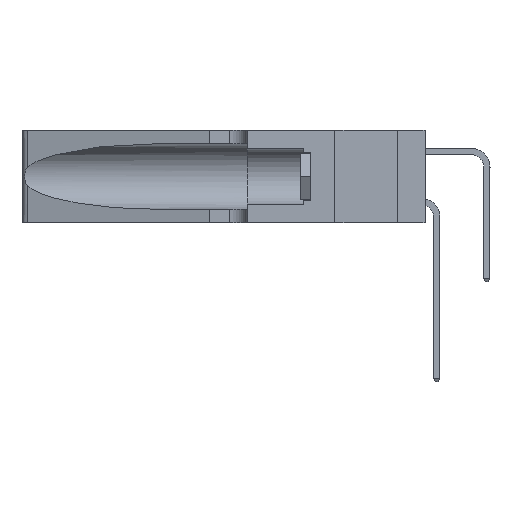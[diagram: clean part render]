
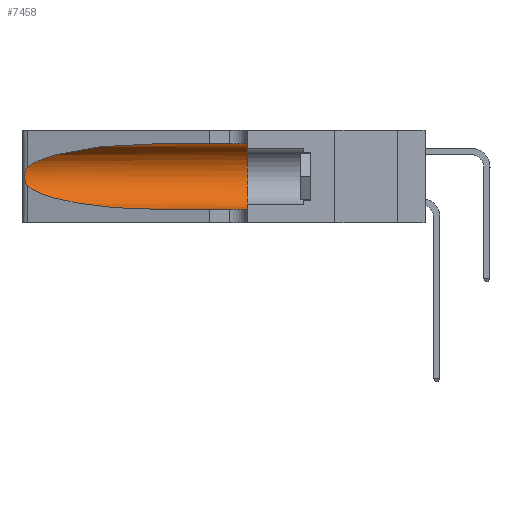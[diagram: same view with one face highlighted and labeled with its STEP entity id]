
A CAD part, left-side view. The second image highlights one B-rep face of the part: STEP entity #7458.
In plain terms, the highlighted cylindrical face has radius 3.308 mm (diameter 6.617 mm), a partial arc.
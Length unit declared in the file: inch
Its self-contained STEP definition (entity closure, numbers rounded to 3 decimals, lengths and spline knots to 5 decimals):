
#196 = AXIS2_PLACEMENT_3D ( 'NONE', #17155, #12661, #23664 ) ;
#1073 = ORIENTED_EDGE ( 'NONE', *, *, #27238, .T. ) ;
#1272 = CARTESIAN_POINT ( 'NONE',  ( 0.1305, 0.72297, 0.05475 ) ) ;
#1434 = LINE ( 'NONE', #25243, #9130 ) ;
#2066 = CARTESIAN_POINT ( 'NONE',  ( 0.25856, 1.23593, 0.16098 ) ) ;
#2228 =( BOUNDED_CURVE ( )  B_SPLINE_CURVE ( 3, ( #24379, #26508, #22404, #5308 ),
 .UNSPECIFIED., .F., .F. ) 
 B_SPLINE_CURVE_WITH_KNOTS ( ( 4, 4 ),
 ( 1.5708, 2.84003 ),
 .UNSPECIFIED. ) 
 CURVE ( )  GEOMETRIC_REPRESENTATION_ITEM ( )  RATIONAL_B_SPLINE_CURVE ( ( 1., 0.87, 0.87, 1. ) ) 
 REPRESENTATION_ITEM ( '' )  );
#2987 = CARTESIAN_POINT ( 'NONE',  ( 0.18966, 0.96281, 0.05475 ) ) ;
#3248 = CARTESIAN_POINT ( 'NONE',  ( 0.1305, 0.72297, 0.31525 ) ) ;
#3663 = ORIENTED_EDGE ( 'NONE', *, *, #13662, .F. ) ;
#3958 = CARTESIAN_POINT ( 'NONE',  ( 0.1305, 0.35, 0.05475 ) ) ;
#4056 = CARTESIAN_POINT ( 'NONE',  ( 0.25487, 1.22718, 0.14631 ) ) ;
#5209 = CARTESIAN_POINT ( 'NONE',  ( 0.25787, 1.23484, 0.2124 ) ) ;
#5308 = CARTESIAN_POINT ( 'NONE',  ( 0.25487, 1.22718, 0.22369 ) ) ;
#6057 = EDGE_CURVE ( 'NONE', #23754, #17033, #24277, .T. ) ;
#6070 = DIRECTION ( 'NONE',  ( 0., -1., 0. ) ) ;
#6397 = CARTESIAN_POINT ( 'NONE',  ( 0.25789, 1.23486, 0.15765 ) ) ;
#6898 = ORIENTED_EDGE ( 'NONE', *, *, #6057, .T. ) ;
#7004 = DIRECTION ( 'NONE',  ( 0., -1., 0. ) ) ;
#7392 = CARTESIAN_POINT ( 'NONE',  ( 0.25487, 1.22718, 0.14631 ) ) ;
#7458 = ADVANCED_FACE ( 'NONE', ( #17317 ), #8222, .F. ) ;
#7813 = LINE ( 'NONE', #25914, #13878 ) ;
#8222 = CYLINDRICAL_SURFACE ( 'NONE', #19831, 0.13025 ) ;
#8605 = EDGE_CURVE ( 'NONE', #17033, #9274, #1434, .T. ) ;
#9130 = VECTOR ( 'NONE', #6070, 39.37008 ) ;
#9274 = VERTEX_POINT ( 'NONE', #3958 ) ;
#9642 = CARTESIAN_POINT ( 'NONE',  ( 0.1305, 0.72297, 0.05475 ) ) ;
#9852 = ORIENTED_EDGE ( 'NONE', *, *, #16700, .T. ) ;
#10794 = CARTESIAN_POINT ( 'NONE',  ( 0.25555, 1.22993, 0.14849 ) ) ;
#10879 = DIRECTION ( 'NONE',  ( 0., -1., 0. ) ) ;
#11335 = B_SPLINE_CURVE_WITH_KNOTS ( 'NONE', 3,
 ( #17562, #21908, #11442, #5209, #20704, #21937, #27174, #23689, #21330, #2066, #6397, #27795, #10794, #4056 ),
 .UNSPECIFIED., .F., .F.,
 ( 4, 2, 2, 2, 2, 2, 4 ),
 ( 0., 0.00027, 0.00053, 0.00107, 0.0016, 0.00187, 0.00214 ),
 .UNSPECIFIED. ) ;
#11442 = CARTESIAN_POINT ( 'NONE',  ( 0.25639, 1.23184, 0.21858 ) ) ;
#12661 = DIRECTION ( 'NONE',  ( 0., 1., 0. ) ) ;
#12931 = VERTEX_POINT ( 'NONE', #3248 ) ;
#13662 = EDGE_CURVE ( 'NONE', #12931, #24186, #7813, .T. ) ;
#13878 = VECTOR ( 'NONE', #10879, 39.37008 ) ;
#14882 = EDGE_LOOP ( 'NONE', ( #1073, #9852, #6898, #20395, #16075, #3663 ) ) ;
#16075 = ORIENTED_EDGE ( 'NONE', *, *, #21393, .F. ) ;
#16700 = EDGE_CURVE ( 'NONE', #22234, #23754, #11335, .T. ) ;
#17033 = VERTEX_POINT ( 'NONE', #1272 ) ;
#17155 = CARTESIAN_POINT ( 'NONE',  ( 0.1305, 0.35, 0.185 ) ) ;
#17317 = FACE_OUTER_BOUND ( 'NONE', #14882, .T. ) ;
#17562 = CARTESIAN_POINT ( 'NONE',  ( 0.25487, 1.22718, 0.22369 ) ) ;
#18111 = CARTESIAN_POINT ( 'NONE',  ( 0.2373, 1.15595, 0.08982 ) ) ;
#18564 = CIRCLE ( 'NONE', #196, 0.13025 ) ;
#19669 = CARTESIAN_POINT ( 'NONE',  ( 0.25487, 1.22718, 0.14631 ) ) ;
#19831 = AXIS2_PLACEMENT_3D ( 'NONE', #26626, #7004, #19957 ) ;
#19957 = DIRECTION ( 'NONE',  ( 0., 0., -1. ) ) ;
#20395 = ORIENTED_EDGE ( 'NONE', *, *, #8605, .T. ) ;
#20704 = CARTESIAN_POINT ( 'NONE',  ( 0.25854, 1.2359, 0.20912 ) ) ;
#21330 = CARTESIAN_POINT ( 'NONE',  ( 0.26017, 1.23833, 0.17102 ) ) ;
#21393 = EDGE_CURVE ( 'NONE', #24186, #9274, #18564, .T. ) ;
#21908 = CARTESIAN_POINT ( 'NONE',  ( 0.25555, 1.22994, 0.2215 ) ) ;
#21937 = CARTESIAN_POINT ( 'NONE',  ( 0.26018, 1.23835, 0.19895 ) ) ;
#22136 = CARTESIAN_POINT ( 'NONE',  ( 0.25487, 1.22718, 0.22369 ) ) ;
#22234 = VERTEX_POINT ( 'NONE', #22136 ) ;
#22404 = CARTESIAN_POINT ( 'NONE',  ( 0.2373, 1.15595, 0.28018 ) ) ;
#23664 = DIRECTION ( 'NONE',  ( 0., 0., 1. ) ) ;
#23689 = CARTESIAN_POINT ( 'NONE',  ( 0.26075, 1.23896, 0.178 ) ) ;
#23754 = VERTEX_POINT ( 'NONE', #19669 ) ;
#24186 = VERTEX_POINT ( 'NONE', #25237 ) ;
#24277 =( BOUNDED_CURVE ( )  B_SPLINE_CURVE ( 3, ( #7392, #18111, #2987, #9642 ),
 .UNSPECIFIED., .F., .T. ) 
 B_SPLINE_CURVE_WITH_KNOTS ( ( 4, 4 ),
 ( 3.44316, 4.71239 ),
 .UNSPECIFIED. ) 
 CURVE ( )  GEOMETRIC_REPRESENTATION_ITEM ( )  RATIONAL_B_SPLINE_CURVE ( ( 1., 0.87, 0.87, 1. ) ) 
 REPRESENTATION_ITEM ( '' )  );
#24379 = CARTESIAN_POINT ( 'NONE',  ( 0.1305, 0.72297, 0.31525 ) ) ;
#25237 = CARTESIAN_POINT ( 'NONE',  ( 0.1305, 0.35, 0.31525 ) ) ;
#25243 = CARTESIAN_POINT ( 'NONE',  ( 0.1305, 1.61858, 0.05475 ) ) ;
#25914 = CARTESIAN_POINT ( 'NONE',  ( 0.1305, 1.61858, 0.31525 ) ) ;
#26508 = CARTESIAN_POINT ( 'NONE',  ( 0.18966, 0.96281, 0.31525 ) ) ;
#26626 = CARTESIAN_POINT ( 'NONE',  ( 0.1305, 1.61858, 0.185 ) ) ;
#27174 = CARTESIAN_POINT ( 'NONE',  ( 0.26075, 1.23896, 0.19203 ) ) ;
#27238 = EDGE_CURVE ( 'NONE', #12931, #22234, #2228, .T. ) ;
#27795 = CARTESIAN_POINT ( 'NONE',  ( 0.25639, 1.23186, 0.15144 ) ) ;
